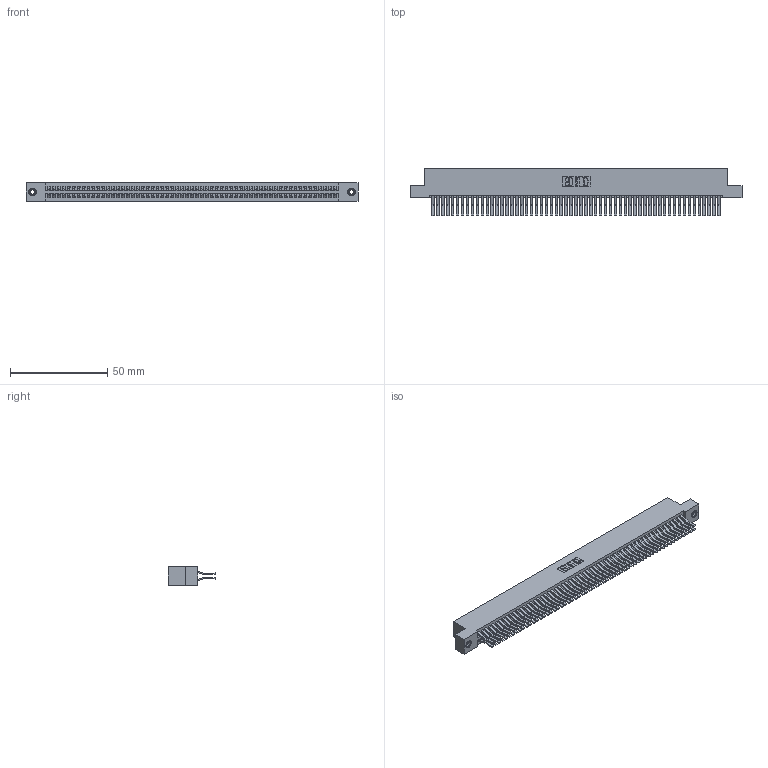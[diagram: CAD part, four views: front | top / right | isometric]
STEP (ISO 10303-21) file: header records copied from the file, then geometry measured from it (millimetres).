
FILE_DESCRIPTION (( 'STEP AP203' ), '1' );
FILE_NAME ('395-118-560-208.STEP', '2019-10-28T03:18:54', ( '' ), ( '' ), 'SwSTEP 2.0', 'SolidWorks 2016', '' );
FILE_SCHEMA (( 'CONFIG_CONTROL_DESIGN' ));
Length unit declared in the file: inch
Products named in the file (4): 345-292-001_560 Tail; 345-250-001_345-250-003-102; 395-118-560-208; 345 Part_Flush Mounting Lugs - 0.156 Dia-TI
Assembly tree (121 placements, depth 2):
  395-118-560-208
    345 Part_Flush Mounting Lugs - 0.156 Dia-TI
    345-292-001_560 Tail  x118
    345-250-001_345-250-003-102  x2
Bounding box: 171.07 x 24.45 x 9.4 mm (x, y, z)
Volume: 17542.5 mm3; surface area: 28262.7 mm2
Topology: 121 solids, 121 shells, 6322 faces, 18767 edges, 12346 vertices
Faces by surface type: plane 4006, cylinder 2300, cone 12, torus 4
Entity records: 45278 total; most frequent: CARTESIAN_POINT 7555, ORIENTED_EDGE 7482, DIRECTION 6671, EDGE_CURVE 3741, LINE 3349, VECTOR 3349, VERTEX_POINT 2488, AXIS2_PLACEMENT_3D 1661
